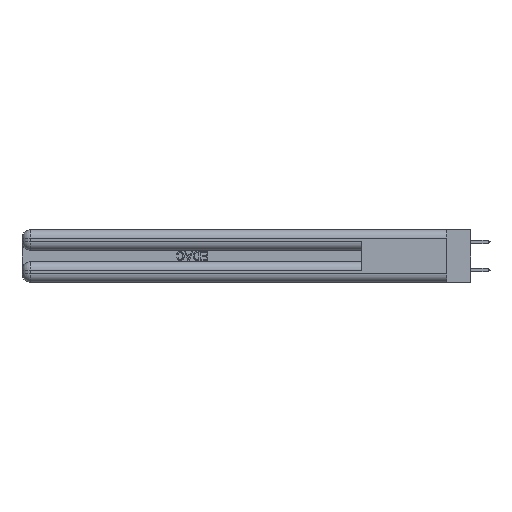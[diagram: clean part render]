
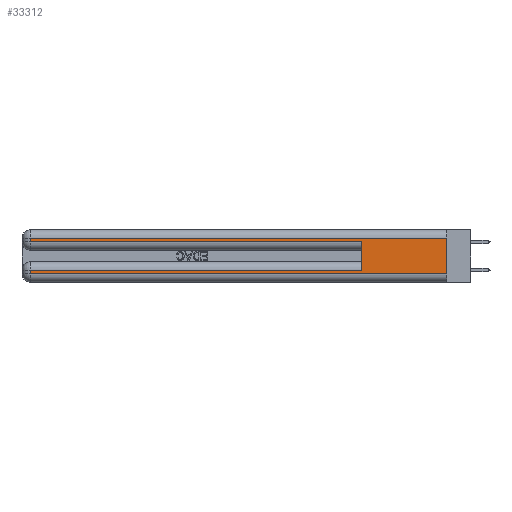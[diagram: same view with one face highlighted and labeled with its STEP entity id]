
A CAD part, left-side view. The second image highlights one B-rep face of the part: STEP entity #33312.
In plain terms, the highlighted planar face has unit normal (-1, 0, 0).
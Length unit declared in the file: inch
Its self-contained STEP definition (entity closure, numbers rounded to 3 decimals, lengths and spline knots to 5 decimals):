
#3898 = VECTOR ( 'NONE', #42247, 39.37008 ) ;
#4100 = EDGE_CURVE ( 'NONE', #31856, #35218, #34783, .T. ) ;
#6236 = VECTOR ( 'NONE', #9407, 39.37008 ) ;
#6520 = ORIENTED_EDGE ( 'NONE', *, *, #43455, .T. ) ;
#7995 = CARTESIAN_POINT ( 'NONE',  ( 0., 2.94, 0.37 ) ) ;
#9286 = EDGE_CURVE ( 'NONE', #12620, #32433, #15998, .T. ) ;
#9407 = DIRECTION ( 'NONE',  ( 0., 0., -1. ) ) ;
#10589 = VECTOR ( 'NONE', #17005, 39.37008 ) ;
#11832 = CARTESIAN_POINT ( 'NONE',  ( 0., 0., 0.37 ) ) ;
#12620 = VERTEX_POINT ( 'NONE', #19769 ) ;
#14402 = CARTESIAN_POINT ( 'NONE',  ( 0., 2.94, 0.285 ) ) ;
#15998 = LINE ( 'NONE', #7995, #22969 ) ;
#16630 = FACE_OUTER_BOUND ( 'NONE', #38083, .T. ) ;
#17005 = DIRECTION ( 'NONE',  ( 0., -1., 0. ) ) ;
#17159 = CARTESIAN_POINT ( 'NONE',  ( 0., 2.94, 0.06 ) ) ;
#17965 = LINE ( 'NONE', #36215, #27104 ) ;
#18345 = CARTESIAN_POINT ( 'NONE',  ( 0., 0., 0.31 ) ) ;
#18835 = DIRECTION ( 'NONE',  ( 0., 0., -1. ) ) ;
#19636 = LINE ( 'NONE', #31528, #10589 ) ;
#19769 = CARTESIAN_POINT ( 'NONE',  ( 0., 2.94, 0.085 ) ) ;
#19790 = DIRECTION ( 'NONE',  ( 0., 0., 1. ) ) ;
#19855 = VECTOR ( 'NONE', #19790, 39.37008 ) ;
#20786 = DIRECTION ( 'NONE',  ( 0., -1., 0. ) ) ;
#21095 = EDGE_CURVE ( 'NONE', #29171, #31508, #27890, .T. ) ;
#21108 = VERTEX_POINT ( 'NONE', #14402 ) ;
#21619 = EDGE_CURVE ( 'NONE', #29171, #12620, #26771, .T. ) ;
#21625 = ORIENTED_EDGE ( 'NONE', *, *, #21095, .F. ) ;
#22498 = DIRECTION ( 'NONE',  ( 0., 0., -1. ) ) ;
#22961 = CARTESIAN_POINT ( 'NONE',  ( 0., 0., 0.06 ) ) ;
#22969 = VECTOR ( 'NONE', #28403, 39.37008 ) ;
#22971 = CARTESIAN_POINT ( 'NONE',  ( 0., 0., 0.37 ) ) ;
#23856 = ORIENTED_EDGE ( 'NONE', *, *, #35536, .T. ) ;
#24220 = CARTESIAN_POINT ( 'NONE',  ( 0., 0., 0.285 ) ) ;
#24847 = ORIENTED_EDGE ( 'NONE', *, *, #21619, .T. ) ;
#26771 = LINE ( 'NONE', #41897, #43847 ) ;
#26857 = VERTEX_POINT ( 'NONE', #22961 ) ;
#27104 = VECTOR ( 'NONE', #22498, 39.37008 ) ;
#27890 = LINE ( 'NONE', #30096, #19855 ) ;
#28270 = ORIENTED_EDGE ( 'NONE', *, *, #38065, .F. ) ;
#28403 = DIRECTION ( 'NONE',  ( 0., 0., -1. ) ) ;
#29171 = VERTEX_POINT ( 'NONE', #30675 ) ;
#29734 = EDGE_CURVE ( 'NONE', #21108, #31508, #41881, .T. ) ;
#30096 = CARTESIAN_POINT ( 'NONE',  ( 0., 0.6, 0.145 ) ) ;
#30675 = CARTESIAN_POINT ( 'NONE',  ( 0., 0.6, 0.085 ) ) ;
#31508 = VERTEX_POINT ( 'NONE', #33367 ) ;
#31528 = CARTESIAN_POINT ( 'NONE',  ( 0., 0., 0.06 ) ) ;
#31856 = VERTEX_POINT ( 'NONE', #34988 ) ;
#32421 = PLANE ( 'NONE',  #37831 ) ;
#32433 = VERTEX_POINT ( 'NONE', #17159 ) ;
#32604 = ORIENTED_EDGE ( 'NONE', *, *, #4100, .T. ) ;
#32810 = VECTOR ( 'NONE', #20786, 39.37008 ) ;
#33312 = ADVANCED_FACE ( 'NONE', ( #16630 ), #32421, .F. ) ;
#33367 = CARTESIAN_POINT ( 'NONE',  ( 0., 0.6, 0.285 ) ) ;
#34783 = LINE ( 'NONE', #18345, #3898 ) ;
#34988 = CARTESIAN_POINT ( 'NONE',  ( 0., 0., 0.31 ) ) ;
#35037 = DIRECTION ( 'NONE',  ( 0., 1., 0. ) ) ;
#35218 = VERTEX_POINT ( 'NONE', #35688 ) ;
#35496 = ORIENTED_EDGE ( 'NONE', *, *, #29734, .T. ) ;
#35536 = EDGE_CURVE ( 'NONE', #32433, #26857, #19636, .T. ) ;
#35688 = CARTESIAN_POINT ( 'NONE',  ( 0., 2.94, 0.31 ) ) ;
#36215 = CARTESIAN_POINT ( 'NONE',  ( 0., 2.94, 0.37 ) ) ;
#36616 = LINE ( 'NONE', #22971, #6236 ) ;
#37831 = AXIS2_PLACEMENT_3D ( 'NONE', #11832, #39288, #18835 ) ;
#38065 = EDGE_CURVE ( 'NONE', #31856, #26857, #36616, .T. ) ;
#38083 = EDGE_LOOP ( 'NONE', ( #28270, #32604, #6520, #35496, #21625, #24847, #42998, #23856 ) ) ;
#39288 = DIRECTION ( 'NONE',  ( 1., 0., 0. ) ) ;
#41881 = LINE ( 'NONE', #24220, #32810 ) ;
#41897 = CARTESIAN_POINT ( 'NONE',  ( 0., 0., 0.085 ) ) ;
#42247 = DIRECTION ( 'NONE',  ( 0., 1., 0. ) ) ;
#42998 = ORIENTED_EDGE ( 'NONE', *, *, #9286, .T. ) ;
#43455 = EDGE_CURVE ( 'NONE', #35218, #21108, #17965, .T. ) ;
#43847 = VECTOR ( 'NONE', #35037, 39.37008 ) ;
